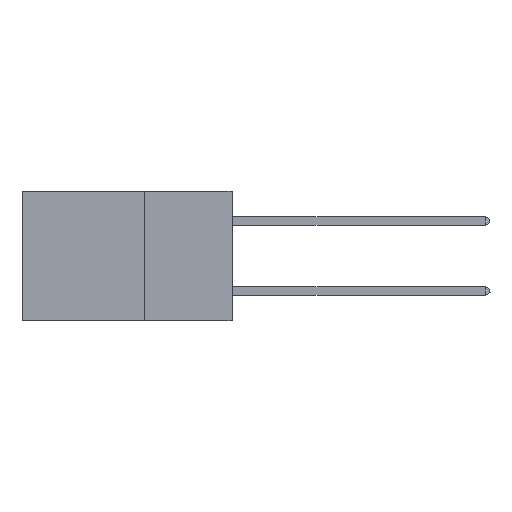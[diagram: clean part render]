
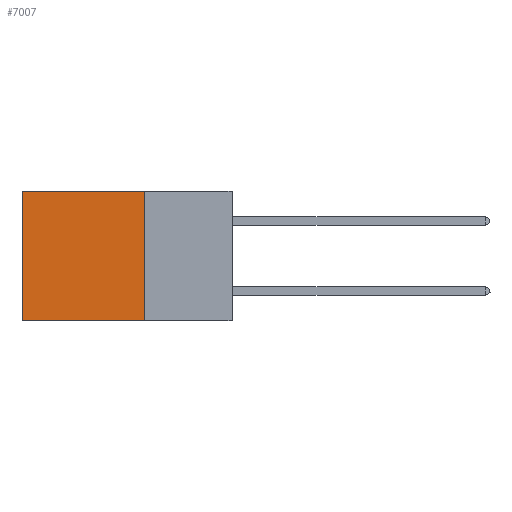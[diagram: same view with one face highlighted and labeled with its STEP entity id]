
A CAD part, left-side view. The second image highlights one B-rep face of the part: STEP entity #7007.
In plain terms, the highlighted planar face has unit normal (-1, 0, 0).
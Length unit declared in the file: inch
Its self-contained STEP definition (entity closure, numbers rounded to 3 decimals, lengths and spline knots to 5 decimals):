
#18 = FACE_OUTER_BOUND ( 'NONE', #15926, .T. ) ;
#107 = DIRECTION ( 'NONE',  ( 0., 0., -1. ) ) ;
#178 = CARTESIAN_POINT ( 'NONE',  ( 0.2875, 0.25, 0. ) ) ;
#218 = VECTOR ( 'NONE', #107, 39.37008 ) ;
#881 = CARTESIAN_POINT ( 'NONE',  ( 0.2875, 0.25, 0. ) ) ;
#1105 = ORIENTED_EDGE ( 'NONE', *, *, #18669, .T. ) ;
#1325 = ORIENTED_EDGE ( 'NONE', *, *, #20840, .T. ) ;
#2528 = EDGE_CURVE ( 'NONE', #11253, #15012, #10355, .T. ) ;
#3292 = LINE ( 'NONE', #15832, #14736 ) ;
#4615 = PLANE ( 'NONE',  #19491 ) ;
#5484 = CARTESIAN_POINT ( 'NONE',  ( 0.2875, 0.6, -0.37 ) ) ;
#6076 = DIRECTION ( 'NONE',  ( 1., 0., 0. ) ) ;
#6223 = LINE ( 'NONE', #20454, #218 ) ;
#6322 = CARTESIAN_POINT ( 'NONE',  ( 0.2875, 0.25, -0.37 ) ) ;
#7007 = ADVANCED_FACE ( 'NONE', ( #18 ), #4615, .F. ) ;
#8034 = VECTOR ( 'NONE', #16502, 39.37008 ) ;
#8349 = VERTEX_POINT ( 'NONE', #5484 ) ;
#9689 = DIRECTION ( 'NONE',  ( 0., 0., -1. ) ) ;
#9805 = CARTESIAN_POINT ( 'NONE',  ( 0.2875, 0.25, -0.37 ) ) ;
#10355 = LINE ( 'NONE', #178, #18501 ) ;
#11253 = VERTEX_POINT ( 'NONE', #16156 ) ;
#12877 = DIRECTION ( 'NONE',  ( 0., 0., -1. ) ) ;
#12932 = LINE ( 'NONE', #6322, #8034 ) ;
#14077 = DIRECTION ( 'NONE',  ( 0., 1., 0. ) ) ;
#14736 = VECTOR ( 'NONE', #14077, 39.37008 ) ;
#14925 = ORIENTED_EDGE ( 'NONE', *, *, #2528, .F. ) ;
#15012 = VERTEX_POINT ( 'NONE', #9805 ) ;
#15821 = VERTEX_POINT ( 'NONE', #18113 ) ;
#15832 = CARTESIAN_POINT ( 'NONE',  ( 0.2875, 0.25, 0. ) ) ;
#15926 = EDGE_LOOP ( 'NONE', ( #1325, #19343, #14925, #1105 ) ) ;
#16156 = CARTESIAN_POINT ( 'NONE',  ( 0.2875, 0.25, 0. ) ) ;
#16502 = DIRECTION ( 'NONE',  ( 0., 1., 0. ) ) ;
#16969 = EDGE_CURVE ( 'NONE', #15012, #8349, #12932, .T. ) ;
#18113 = CARTESIAN_POINT ( 'NONE',  ( 0.2875, 0.6, 0. ) ) ;
#18501 = VECTOR ( 'NONE', #12877, 39.37008 ) ;
#18669 = EDGE_CURVE ( 'NONE', #11253, #15821, #3292, .T. ) ;
#19343 = ORIENTED_EDGE ( 'NONE', *, *, #16969, .F. ) ;
#19491 = AXIS2_PLACEMENT_3D ( 'NONE', #881, #6076, #9689 ) ;
#20454 = CARTESIAN_POINT ( 'NONE',  ( 0.2875, 0.6, 0. ) ) ;
#20840 = EDGE_CURVE ( 'NONE', #15821, #8349, #6223, .T. ) ;
